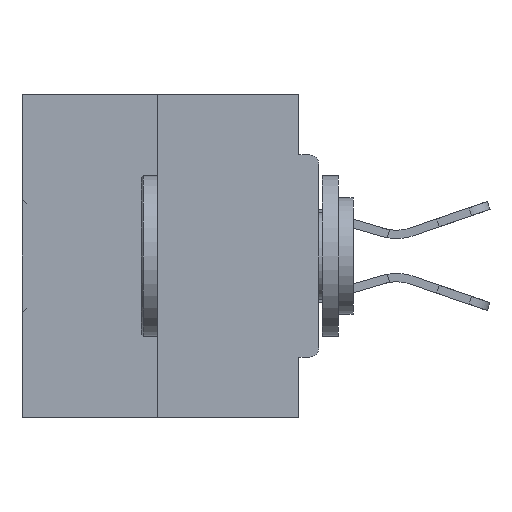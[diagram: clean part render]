
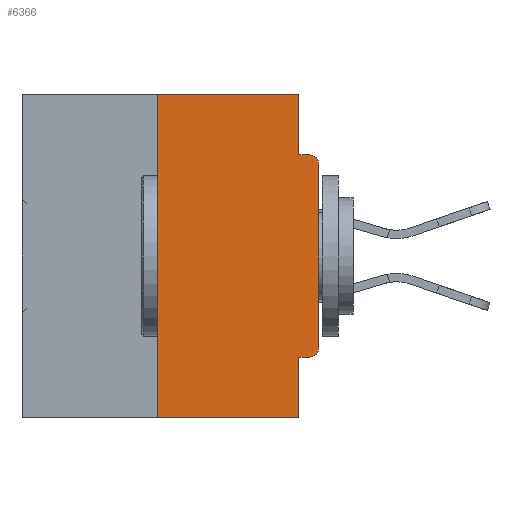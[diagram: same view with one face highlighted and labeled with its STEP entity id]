
A CAD part, left-side view. The second image highlights one B-rep face of the part: STEP entity #6366.
In plain terms, the highlighted planar face has unit normal (-1, 0, 0).
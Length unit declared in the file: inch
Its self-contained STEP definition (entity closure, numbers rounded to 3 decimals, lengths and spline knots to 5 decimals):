
#2040 = EDGE_CURVE ( 'NONE', #38270, #10333, #8909, .T. ) ;
#2961 = VERTEX_POINT ( 'NONE', #24412 ) ;
#3182 = LINE ( 'NONE', #33230, #30441 ) ;
#3822 = DIRECTION ( 'NONE',  ( 0., 0., 1. ) ) ;
#4881 = LINE ( 'NONE', #46489, #11277 ) ;
#5728 = ORIENTED_EDGE ( 'NONE', *, *, #42994, .T. ) ;
#6366 = ADVANCED_FACE ( 'NONE', ( #36100 ), #46835, .F. ) ;
#6954 = ORIENTED_EDGE ( 'NONE', *, *, #15390, .F. ) ;
#8326 = ORIENTED_EDGE ( 'NONE', *, *, #17335, .F. ) ;
#8909 = LINE ( 'NONE', #16521, #10089 ) ;
#9110 = EDGE_CURVE ( 'NONE', #38270, #25599, #28917, .T. ) ;
#9371 = ORIENTED_EDGE ( 'NONE', *, *, #46152, .F. ) ;
#9896 = DIRECTION ( 'NONE',  ( 0., 1., 0. ) ) ;
#10089 = VECTOR ( 'NONE', #38583, 39.37008 ) ;
#10333 = VERTEX_POINT ( 'NONE', #23677 ) ;
#11277 = VECTOR ( 'NONE', #38986, 39.37008 ) ;
#11541 = CARTESIAN_POINT ( 'NONE',  ( 0., 0., -0.1085 ) ) ;
#11558 = CARTESIAN_POINT ( 'NONE',  ( 0., 0., -0.0935 ) ) ;
#11974 = CARTESIAN_POINT ( 'NONE',  ( 0., 0.015, -0.0935 ) ) ;
#12913 = AXIS2_PLACEMENT_3D ( 'NONE', #42930, #39503, #24773 ) ;
#13214 = DIRECTION ( 'NONE',  ( 0., -1., 0. ) ) ;
#13225 = EDGE_CURVE ( 'NONE', #2961, #47021, #42164, .T. ) ;
#14042 = DIRECTION ( 'NONE',  ( -1., 0., 0. ) ) ;
#14383 = DIRECTION ( 'NONE',  ( 0., 0., -1. ) ) ;
#15390 = EDGE_CURVE ( 'NONE', #10333, #25579, #4881, .T. ) ;
#16521 = CARTESIAN_POINT ( 'NONE',  ( 0., 0.25, 0. ) ) ;
#17335 = EDGE_CURVE ( 'NONE', #27448, #44573, #27791, .T. ) ;
#18675 = DIRECTION ( 'NONE',  ( -1., 0., 0. ) ) ;
#19304 = DIRECTION ( 'NONE',  ( 0., 0., -1. ) ) ;
#19959 = CARTESIAN_POINT ( 'NONE',  ( 0., 0.015, -0.4065 ) ) ;
#20597 = VERTEX_POINT ( 'NONE', #19959 ) ;
#20618 = LINE ( 'NONE', #36850, #43867 ) ;
#21283 = ORIENTED_EDGE ( 'NONE', *, *, #9110, .T. ) ;
#21565 = CARTESIAN_POINT ( 'NONE',  ( 0., 0., -0.4065 ) ) ;
#22749 = EDGE_CURVE ( 'NONE', #20597, #2961, #28921, .T. ) ;
#23476 = CARTESIAN_POINT ( 'NONE',  ( 0., 0.031, -0.5 ) ) ;
#23677 = CARTESIAN_POINT ( 'NONE',  ( 0., 0.25, 0. ) ) ;
#24412 = CARTESIAN_POINT ( 'NONE',  ( 0., 0., -0.3915 ) ) ;
#24773 = DIRECTION ( 'NONE',  ( 0., 0., -1. ) ) ;
#25579 = VERTEX_POINT ( 'NONE', #37907 ) ;
#25599 = VERTEX_POINT ( 'NONE', #23476 ) ;
#25797 = VECTOR ( 'NONE', #9896, 39.37008 ) ;
#26018 = CARTESIAN_POINT ( 'NONE',  ( 0., 0.015, -0.1085 ) ) ;
#26553 = VERTEX_POINT ( 'NONE', #42760 ) ;
#27448 = VERTEX_POINT ( 'NONE', #44321 ) ;
#27791 = LINE ( 'NONE', #11558, #46928 ) ;
#27887 = EDGE_CURVE ( 'NONE', #20597, #26553, #35613, .T. ) ;
#28917 = LINE ( 'NONE', #32534, #32357 ) ;
#28921 = CIRCLE ( 'NONE', #47887, 0.015 ) ;
#29775 = ORIENTED_EDGE ( 'NONE', *, *, #27887, .F. ) ;
#30086 = DIRECTION ( 'NONE',  ( 0., -1., 0. ) ) ;
#30441 = VECTOR ( 'NONE', #14383, 39.37008 ) ;
#31831 = ORIENTED_EDGE ( 'NONE', *, *, #39859, .F. ) ;
#32329 = VECTOR ( 'NONE', #3822, 39.37008 ) ;
#32357 = VECTOR ( 'NONE', #13214, 39.37008 ) ;
#32534 = CARTESIAN_POINT ( 'NONE',  ( 0., 0.46, -0.5 ) ) ;
#33230 = CARTESIAN_POINT ( 'NONE',  ( 0., 0.031, -0.5 ) ) ;
#33447 = DIRECTION ( 'NONE',  ( 0., 0., -1. ) ) ;
#35613 = LINE ( 'NONE', #21565, #25797 ) ;
#35635 = ORIENTED_EDGE ( 'NONE', *, *, #13225, .T. ) ;
#36100 = FACE_OUTER_BOUND ( 'NONE', #43658, .T. ) ;
#36616 = DIRECTION ( 'NONE',  ( 0., 0., -1. ) ) ;
#36850 = CARTESIAN_POINT ( 'NONE',  ( 0., 0.031, 0. ) ) ;
#37907 = CARTESIAN_POINT ( 'NONE',  ( 0., 0.031, 0. ) ) ;
#38270 = VERTEX_POINT ( 'NONE', #45083 ) ;
#38583 = DIRECTION ( 'NONE',  ( 0., 0., 1. ) ) ;
#38986 = DIRECTION ( 'NONE',  ( 0., -1., 0. ) ) ;
#39110 = ORIENTED_EDGE ( 'NONE', *, *, #2040, .F. ) ;
#39503 = DIRECTION ( 'NONE',  ( 1., 0., 0. ) ) ;
#39859 = EDGE_CURVE ( 'NONE', #26553, #25599, #3182, .T. ) ;
#41126 = CARTESIAN_POINT ( 'NONE',  ( 0., 0., 0. ) ) ;
#42164 = LINE ( 'NONE', #41126, #32329 ) ;
#42760 = CARTESIAN_POINT ( 'NONE',  ( 0., 0.031, -0.4065 ) ) ;
#42930 = CARTESIAN_POINT ( 'NONE',  ( 0., 0.46, 0. ) ) ;
#42994 = EDGE_CURVE ( 'NONE', #47021, #44573, #46423, .T. ) ;
#43513 = AXIS2_PLACEMENT_3D ( 'NONE', #26018, #18675, #19304 ) ;
#43658 = EDGE_LOOP ( 'NONE', ( #6954, #39110, #21283, #31831, #29775, #46641, #35635, #5728, #8326, #9371 ) ) ;
#43867 = VECTOR ( 'NONE', #33447, 39.37008 ) ;
#44321 = CARTESIAN_POINT ( 'NONE',  ( 0., 0.031, -0.0935 ) ) ;
#44573 = VERTEX_POINT ( 'NONE', #11974 ) ;
#45083 = CARTESIAN_POINT ( 'NONE',  ( 0., 0.25, -0.5 ) ) ;
#46152 = EDGE_CURVE ( 'NONE', #25579, #27448, #20618, .T. ) ;
#46423 = CIRCLE ( 'NONE', #43513, 0.015 ) ;
#46489 = CARTESIAN_POINT ( 'NONE',  ( 0., 0.46, 0. ) ) ;
#46641 = ORIENTED_EDGE ( 'NONE', *, *, #22749, .T. ) ;
#46835 = PLANE ( 'NONE',  #12913 ) ;
#46928 = VECTOR ( 'NONE', #30086, 39.37008 ) ;
#47021 = VERTEX_POINT ( 'NONE', #11541 ) ;
#47832 = CARTESIAN_POINT ( 'NONE',  ( 0., 0.015, -0.3915 ) ) ;
#47887 = AXIS2_PLACEMENT_3D ( 'NONE', #47832, #14042, #36616 ) ;
